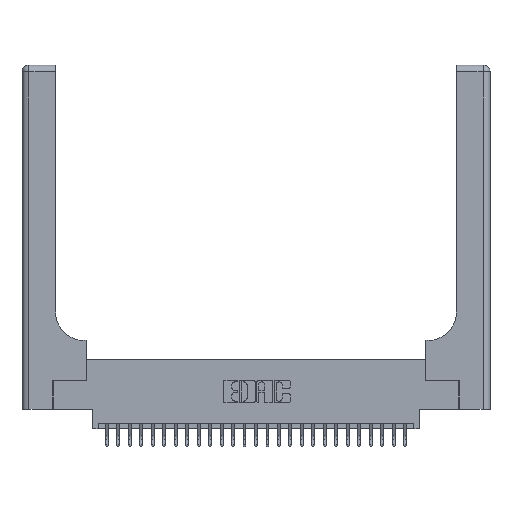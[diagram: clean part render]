
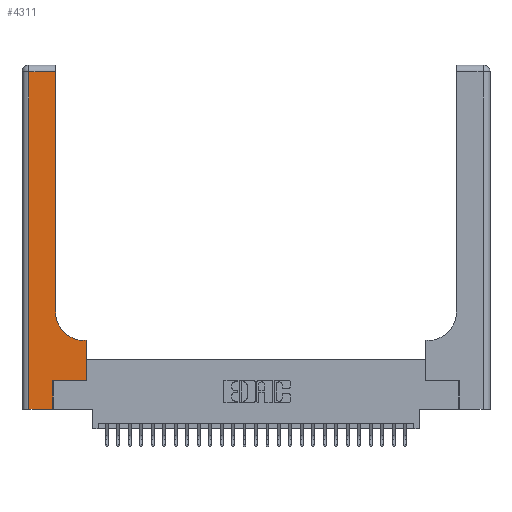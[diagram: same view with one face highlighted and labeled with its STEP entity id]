
A CAD part, top view. The second image highlights one B-rep face of the part: STEP entity #4311.
In plain terms, the highlighted planar face has unit normal (0, 0, 1).
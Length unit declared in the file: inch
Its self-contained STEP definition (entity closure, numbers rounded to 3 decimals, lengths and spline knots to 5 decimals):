
#1875 = CIRCLE ( 'NONE', #7144, 0.25 ) ;
#2154 = CARTESIAN_POINT ( 'NONE',  ( 0., 2.94, 0.37 ) ) ;
#2229 = VECTOR ( 'NONE', #28072, 39.37008 ) ;
#2904 = LINE ( 'NONE', #25873, #2229 ) ;
#3274 = LINE ( 'NONE', #18407, #7845 ) ;
#3524 = ORIENTED_EDGE ( 'NONE', *, *, #25980, .T. ) ;
#4311 = ADVANCED_FACE ( 'NONE', ( #20239 ), #15658, .F. ) ;
#4395 = CARTESIAN_POINT ( 'NONE',  ( 0.06, 0., 0.37 ) ) ;
#4476 = DIRECTION ( 'NONE',  ( -1., 0., 0. ) ) ;
#6098 = CARTESIAN_POINT ( 'NONE',  ( 0.269, 0., 0.37 ) ) ;
#6279 = CARTESIAN_POINT ( 'NONE',  ( 0.5415, 0.85, 0.37 ) ) ;
#6847 = EDGE_LOOP ( 'NONE', ( #20281, #22727, #17252, #24176, #26421, #3524, #21823, #7737, #19136 ) ) ;
#7048 = AXIS2_PLACEMENT_3D ( 'NONE', #22369, #26806, #13538 ) ;
#7144 = AXIS2_PLACEMENT_3D ( 'NONE', #6279, #21796, #8559 ) ;
#7407 = VERTEX_POINT ( 'NONE', #21082 ) ;
#7737 = ORIENTED_EDGE ( 'NONE', *, *, #7905, .T. ) ;
#7845 = VECTOR ( 'NONE', #20565, 39.37008 ) ;
#7905 = EDGE_CURVE ( 'NONE', #26301, #19652, #22497, .T. ) ;
#8559 = DIRECTION ( 'NONE',  ( 1., 0., 0. ) ) ;
#9181 = VERTEX_POINT ( 'NONE', #4395 ) ;
#9689 = LINE ( 'NONE', #6098, #20756 ) ;
#10057 = VECTOR ( 'NONE', #4476, 39.37008 ) ;
#10517 = CARTESIAN_POINT ( 'NONE',  ( 0., 0., 0.37 ) ) ;
#10606 = DIRECTION ( 'NONE',  ( 0., 1., 0. ) ) ;
#10779 = CARTESIAN_POINT ( 'NONE',  ( 0.5415, 0.6, 0.37 ) ) ;
#11802 = CARTESIAN_POINT ( 'NONE',  ( 0.2915, 3., 0.37 ) ) ;
#12058 = EDGE_CURVE ( 'NONE', #24110, #7407, #17603, .T. ) ;
#12425 = VECTOR ( 'NONE', #15445, 39.37008 ) ;
#12444 = CARTESIAN_POINT ( 'NONE',  ( 0.5585, 0.25, 0.37 ) ) ;
#13538 = DIRECTION ( 'NONE',  ( -1., 0., 0. ) ) ;
#13592 = EDGE_CURVE ( 'NONE', #7407, #9181, #2904, .T. ) ;
#13650 = CARTESIAN_POINT ( 'NONE',  ( 0.269, 0., 0.37 ) ) ;
#13924 = VERTEX_POINT ( 'NONE', #13650 ) ;
#14638 = DIRECTION ( 'NONE',  ( 0., 1., 0. ) ) ;
#14937 = CARTESIAN_POINT ( 'NONE',  ( 0.2915, 0.85, 0.37 ) ) ;
#14961 = VERTEX_POINT ( 'NONE', #14937 ) ;
#15445 = DIRECTION ( 'NONE',  ( -1., 0., 0. ) ) ;
#15611 = EDGE_CURVE ( 'NONE', #13924, #20009, #9689, .T. ) ;
#15658 = PLANE ( 'NONE',  #7048 ) ;
#15780 = EDGE_CURVE ( 'NONE', #9181, #13924, #21798, .T. ) ;
#15870 = VECTOR ( 'NONE', #26721, 39.37008 ) ;
#16533 = VERTEX_POINT ( 'NONE', #19046 ) ;
#17252 = ORIENTED_EDGE ( 'NONE', *, *, #13592, .T. ) ;
#17603 = LINE ( 'NONE', #2154, #12425 ) ;
#17705 = EDGE_CURVE ( 'NONE', #19652, #14961, #1875, .T. ) ;
#18041 = EDGE_CURVE ( 'NONE', #14961, #24110, #28208, .T. ) ;
#18407 = CARTESIAN_POINT ( 'NONE',  ( 0.269, 0.25, 0.37 ) ) ;
#18768 = EDGE_CURVE ( 'NONE', #16533, #26301, #22642, .T. ) ;
#19046 = CARTESIAN_POINT ( 'NONE',  ( 0.5585, 0.25, 0.37 ) ) ;
#19136 = ORIENTED_EDGE ( 'NONE', *, *, #17705, .T. ) ;
#19652 = VERTEX_POINT ( 'NONE', #10779 ) ;
#20009 = VERTEX_POINT ( 'NONE', #20692 ) ;
#20239 = FACE_OUTER_BOUND ( 'NONE', #6847, .T. ) ;
#20281 = ORIENTED_EDGE ( 'NONE', *, *, #18041, .T. ) ;
#20565 = DIRECTION ( 'NONE',  ( 1., 0., 0. ) ) ;
#20692 = CARTESIAN_POINT ( 'NONE',  ( 0.269, 0.25, 0.37 ) ) ;
#20756 = VECTOR ( 'NONE', #10606, 39.37008 ) ;
#21082 = CARTESIAN_POINT ( 'NONE',  ( 0.06, 2.94, 0.37 ) ) ;
#21796 = DIRECTION ( 'NONE',  ( 0., 0., -1. ) ) ;
#21798 = LINE ( 'NONE', #10517, #15870 ) ;
#21823 = ORIENTED_EDGE ( 'NONE', *, *, #18768, .T. ) ;
#22353 = VECTOR ( 'NONE', #25040, 39.37008 ) ;
#22369 = CARTESIAN_POINT ( 'NONE',  ( 0., 3., 0.37 ) ) ;
#22497 = LINE ( 'NONE', #24427, #10057 ) ;
#22642 = LINE ( 'NONE', #12444, #27819 ) ;
#22727 = ORIENTED_EDGE ( 'NONE', *, *, #12058, .T. ) ;
#23848 = CARTESIAN_POINT ( 'NONE',  ( 0.2915, 2.94, 0.37 ) ) ;
#23938 = CARTESIAN_POINT ( 'NONE',  ( 0.5585, 0.6, 0.37 ) ) ;
#24110 = VERTEX_POINT ( 'NONE', #23848 ) ;
#24176 = ORIENTED_EDGE ( 'NONE', *, *, #15780, .T. ) ;
#24427 = CARTESIAN_POINT ( 'NONE',  ( 0.2915, 0.6, 0.37 ) ) ;
#25040 = DIRECTION ( 'NONE',  ( 0., 1., 0. ) ) ;
#25873 = CARTESIAN_POINT ( 'NONE',  ( 0.06, 3., 0.37 ) ) ;
#25980 = EDGE_CURVE ( 'NONE', #20009, #16533, #3274, .T. ) ;
#26301 = VERTEX_POINT ( 'NONE', #23938 ) ;
#26421 = ORIENTED_EDGE ( 'NONE', *, *, #15611, .T. ) ;
#26721 = DIRECTION ( 'NONE',  ( 1., 0., 0. ) ) ;
#26806 = DIRECTION ( 'NONE',  ( 0., 0., -1. ) ) ;
#27819 = VECTOR ( 'NONE', #14638, 39.37008 ) ;
#28072 = DIRECTION ( 'NONE',  ( 0., -1., 0. ) ) ;
#28208 = LINE ( 'NONE', #11802, #22353 ) ;
